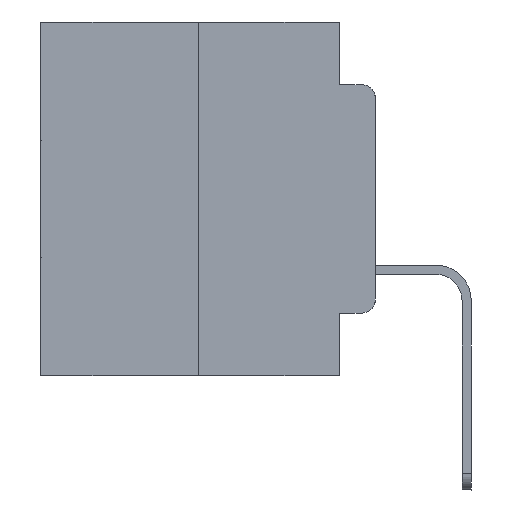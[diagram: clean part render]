
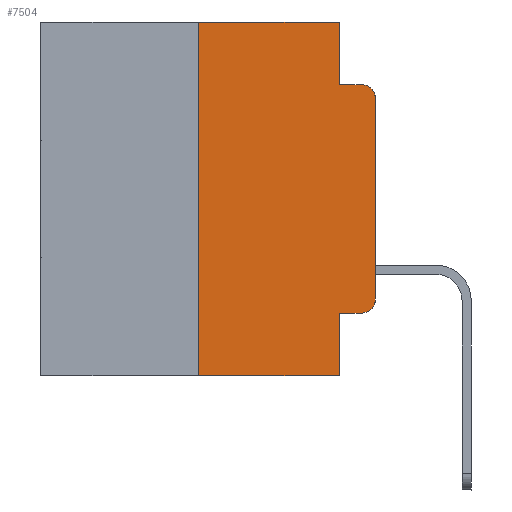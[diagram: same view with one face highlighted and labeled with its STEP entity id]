
A CAD part, left-side view. The second image highlights one B-rep face of the part: STEP entity #7504.
In plain terms, the highlighted planar face has unit normal (-1, 0, 0).
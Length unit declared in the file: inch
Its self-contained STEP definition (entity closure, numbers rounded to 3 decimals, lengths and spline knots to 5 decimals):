
#19 = EDGE_CURVE ( 'NONE', #11221, #24660, #18795, .T. ) ;
#194 = EDGE_CURVE ( 'NONE', #3509, #5228, #5409, .T. ) ;
#308 = CARTESIAN_POINT ( 'NONE',  ( 0., 0.051, -0.0885 ) ) ;
#1049 = ORIENTED_EDGE ( 'NONE', *, *, #194, .F. ) ;
#1509 = VERTEX_POINT ( 'NONE', #26236 ) ;
#1616 = CARTESIAN_POINT ( 'NONE',  ( 0., 0.051, 0. ) ) ;
#2381 = VECTOR ( 'NONE', #16544, 39.37008 ) ;
#2823 = VERTEX_POINT ( 'NONE', #23786 ) ;
#2842 = CARTESIAN_POINT ( 'NONE',  ( 0., 0.25, -0.5 ) ) ;
#2962 = VECTOR ( 'NONE', #21039, 39.37008 ) ;
#3058 = EDGE_LOOP ( 'NONE', ( #8137, #13055, #1049, #9838, #14912, #4360, #7879, #7197, #11979, #14549 ) ) ;
#3242 = VERTEX_POINT ( 'NONE', #12268 ) ;
#3509 = VERTEX_POINT ( 'NONE', #308 ) ;
#3523 = DIRECTION ( 'NONE',  ( 0., 0., -1. ) ) ;
#4000 = LINE ( 'NONE', #1616, #2962 ) ;
#4199 = DIRECTION ( 'NONE',  ( 0., -1., 0. ) ) ;
#4320 = CARTESIAN_POINT ( 'NONE',  ( 0., 0.051, -0.0885 ) ) ;
#4360 = ORIENTED_EDGE ( 'NONE', *, *, #20135, .F. ) ;
#4954 = VERTEX_POINT ( 'NONE', #2842 ) ;
#5096 = CARTESIAN_POINT ( 'NONE',  ( 0., 0.02, -0.3915 ) ) ;
#5110 = CARTESIAN_POINT ( 'NONE',  ( 0., 0.25, 0. ) ) ;
#5228 = VERTEX_POINT ( 'NONE', #23077 ) ;
#5409 = LINE ( 'NONE', #4320, #26501 ) ;
#5486 = VERTEX_POINT ( 'NONE', #15719 ) ;
#5781 = EDGE_CURVE ( 'NONE', #1509, #2823, #15677, .T. ) ;
#7197 = ORIENTED_EDGE ( 'NONE', *, *, #18965, .F. ) ;
#7504 = ADVANCED_FACE ( 'NONE', ( #7530 ), #20939, .F. ) ;
#7530 = FACE_OUTER_BOUND ( 'NONE', #3058, .T. ) ;
#7879 = ORIENTED_EDGE ( 'NONE', *, *, #13600, .T. ) ;
#8061 = VERTEX_POINT ( 'NONE', #19224 ) ;
#8137 = ORIENTED_EDGE ( 'NONE', *, *, #9383, .T. ) ;
#8149 = CIRCLE ( 'NONE', #13663, 0.02 ) ;
#8472 = EDGE_CURVE ( 'NONE', #8061, #5228, #8149, .T. ) ;
#9226 = AXIS2_PLACEMENT_3D ( 'NONE', #5096, #17776, #24138 ) ;
#9383 = EDGE_CURVE ( 'NONE', #3242, #8061, #18414, .T. ) ;
#9838 = ORIENTED_EDGE ( 'NONE', *, *, #17340, .F. ) ;
#9862 = CIRCLE ( 'NONE', #9226, 0.02 ) ;
#10063 = DIRECTION ( 'NONE',  ( 0., -1., 0. ) ) ;
#10561 = CARTESIAN_POINT ( 'NONE',  ( 0., 0., 0. ) ) ;
#11221 = VERTEX_POINT ( 'NONE', #5110 ) ;
#11979 = ORIENTED_EDGE ( 'NONE', *, *, #5781, .T. ) ;
#12268 = CARTESIAN_POINT ( 'NONE',  ( 0., 0., -0.3915 ) ) ;
#12669 = CARTESIAN_POINT ( 'NONE',  ( 0., 0.051, -0.4115 ) ) ;
#12787 = DIRECTION ( 'NONE',  ( 0., 0., 1. ) ) ;
#12798 = LINE ( 'NONE', #20372, #13849 ) ;
#13055 = ORIENTED_EDGE ( 'NONE', *, *, #8472, .T. ) ;
#13600 = EDGE_CURVE ( 'NONE', #4954, #5486, #12798, .T. ) ;
#13663 = AXIS2_PLACEMENT_3D ( 'NONE', #20429, #22649, #3523 ) ;
#13849 = VECTOR ( 'NONE', #10063, 39.37008 ) ;
#14549 = ORIENTED_EDGE ( 'NONE', *, *, #20581, .T. ) ;
#14785 = DIRECTION ( 'NONE',  ( 1., 0., 0. ) ) ;
#14912 = ORIENTED_EDGE ( 'NONE', *, *, #19, .F. ) ;
#15164 = DIRECTION ( 'NONE',  ( 0., -1., 0. ) ) ;
#15677 = LINE ( 'NONE', #12669, #27705 ) ;
#15719 = CARTESIAN_POINT ( 'NONE',  ( 0., 0.051, -0.5 ) ) ;
#16544 = DIRECTION ( 'NONE',  ( 0., 0., -1. ) ) ;
#17097 = VECTOR ( 'NONE', #12787, 39.37008 ) ;
#17340 = EDGE_CURVE ( 'NONE', #24660, #3509, #25819, .T. ) ;
#17776 = DIRECTION ( 'NONE',  ( -1., 0., 0. ) ) ;
#17998 = DIRECTION ( 'NONE',  ( 0., 0., 1. ) ) ;
#18414 = LINE ( 'NONE', #10561, #17097 ) ;
#18795 = LINE ( 'NONE', #27538, #25506 ) ;
#18904 = CARTESIAN_POINT ( 'NONE',  ( 0., 0.051, 0. ) ) ;
#18965 = EDGE_CURVE ( 'NONE', #1509, #5486, #4000, .T. ) ;
#19149 = DIRECTION ( 'NONE',  ( 0., 0., -1. ) ) ;
#19224 = CARTESIAN_POINT ( 'NONE',  ( 0., 0., -0.1085 ) ) ;
#19266 = VECTOR ( 'NONE', #17998, 39.37008 ) ;
#20135 = EDGE_CURVE ( 'NONE', #4954, #11221, #24286, .T. ) ;
#20372 = CARTESIAN_POINT ( 'NONE',  ( 0., 0.473, -0.5 ) ) ;
#20429 = CARTESIAN_POINT ( 'NONE',  ( 0., 0.02, -0.1085 ) ) ;
#20581 = EDGE_CURVE ( 'NONE', #2823, #3242, #9862, .T. ) ;
#20939 = PLANE ( 'NONE',  #20984 ) ;
#20984 = AXIS2_PLACEMENT_3D ( 'NONE', #21206, #14785, #19149 ) ;
#21039 = DIRECTION ( 'NONE',  ( 0., 0., -1. ) ) ;
#21206 = CARTESIAN_POINT ( 'NONE',  ( 0., 0.473, 0. ) ) ;
#22563 = CARTESIAN_POINT ( 'NONE',  ( 0., 0.25, 0. ) ) ;
#22649 = DIRECTION ( 'NONE',  ( -1., 0., 0. ) ) ;
#23077 = CARTESIAN_POINT ( 'NONE',  ( 0., 0.02, -0.0885 ) ) ;
#23786 = CARTESIAN_POINT ( 'NONE',  ( 0., 0.02, -0.4115 ) ) ;
#24138 = DIRECTION ( 'NONE',  ( 0., 0., -1. ) ) ;
#24286 = LINE ( 'NONE', #22563, #19266 ) ;
#24660 = VERTEX_POINT ( 'NONE', #18904 ) ;
#25045 = CARTESIAN_POINT ( 'NONE',  ( 0., 0.051, 0. ) ) ;
#25492 = DIRECTION ( 'NONE',  ( 0., -1., 0. ) ) ;
#25506 = VECTOR ( 'NONE', #25492, 39.37008 ) ;
#25819 = LINE ( 'NONE', #25045, #2381 ) ;
#26236 = CARTESIAN_POINT ( 'NONE',  ( 0., 0.051, -0.4115 ) ) ;
#26501 = VECTOR ( 'NONE', #15164, 39.37008 ) ;
#27538 = CARTESIAN_POINT ( 'NONE',  ( 0., 0.473, 0. ) ) ;
#27705 = VECTOR ( 'NONE', #4199, 39.37008 ) ;
